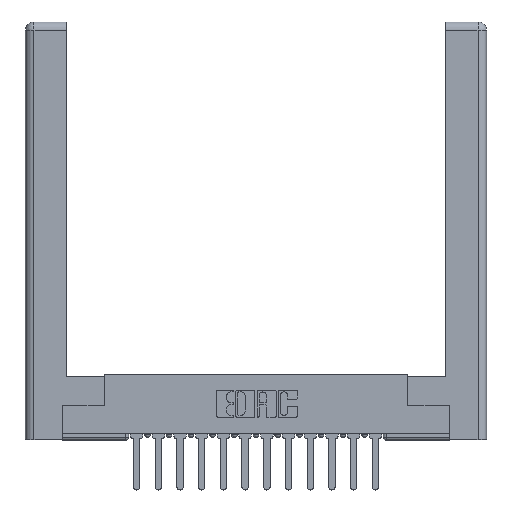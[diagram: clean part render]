
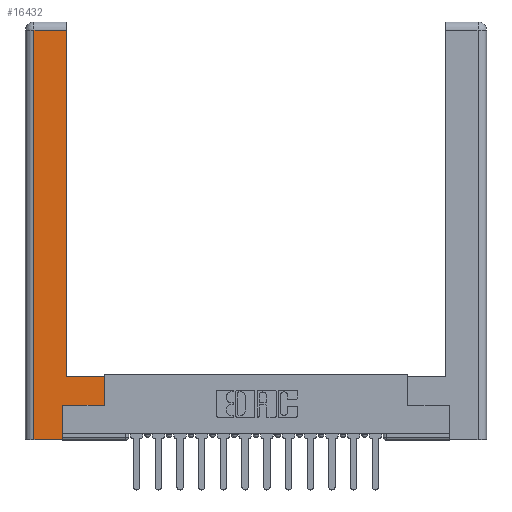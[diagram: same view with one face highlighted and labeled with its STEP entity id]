
A CAD part, top view. The second image highlights one B-rep face of the part: STEP entity #16432.
In plain terms, the highlighted planar face has unit normal (0, 0, 1).
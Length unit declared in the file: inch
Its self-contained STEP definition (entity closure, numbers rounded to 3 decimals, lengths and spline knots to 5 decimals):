
#185 = VECTOR ( 'NONE', #12229, 39.37008 ) ;
#462 = CARTESIAN_POINT ( 'NONE',  ( 0.295, 3., 0. ) ) ;
#764 = VECTOR ( 'NONE', #3290, 39.37008 ) ;
#845 = CARTESIAN_POINT ( 'NONE',  ( 0.265, 0., 0. ) ) ;
#941 = EDGE_CURVE ( 'NONE', #9943, #2166, #15831, .T. ) ;
#943 = ORIENTED_EDGE ( 'NONE', *, *, #9176, .T. ) ;
#1061 = FACE_OUTER_BOUND ( 'NONE', #15952, .T. ) ;
#1888 = DIRECTION ( 'NONE',  ( 0., 1., 0. ) ) ;
#2166 = VERTEX_POINT ( 'NONE', #6446 ) ;
#2201 = LINE ( 'NONE', #7505, #14871 ) ;
#2203 = EDGE_CURVE ( 'NONE', #6351, #10441, #2510, .T. ) ;
#2479 = VECTOR ( 'NONE', #5366, 39.37008 ) ;
#2510 = LINE ( 'NONE', #2670, #2479 ) ;
#2670 = CARTESIAN_POINT ( 'NONE',  ( 0.0615, 0., 0. ) ) ;
#2822 = CARTESIAN_POINT ( 'NONE',  ( 0.0615, 2.94, 0. ) ) ;
#2996 = DIRECTION ( 'NONE',  ( 0., 1., 0. ) ) ;
#3290 = DIRECTION ( 'NONE',  ( 0., 1., 0. ) ) ;
#3300 = EDGE_CURVE ( 'NONE', #8840, #8304, #14601, .T. ) ;
#4397 = EDGE_CURVE ( 'NONE', #10441, #9943, #16046, .T. ) ;
#4528 = CARTESIAN_POINT ( 'NONE',  ( 0.265, 0.245, 0. ) ) ;
#4725 = CARTESIAN_POINT ( 'NONE',  ( 0.565, 0.245, 0. ) ) ;
#5174 = ORIENTED_EDGE ( 'NONE', *, *, #941, .T. ) ;
#5181 = DIRECTION ( 'NONE',  ( -1., 0., 0. ) ) ;
#5227 = ORIENTED_EDGE ( 'NONE', *, *, #2203, .T. ) ;
#5366 = DIRECTION ( 'NONE',  ( 0., -1., 0. ) ) ;
#5504 = VECTOR ( 'NONE', #2996, 39.37008 ) ;
#5516 = CARTESIAN_POINT ( 'NONE',  ( 0.565, 0.45, 0. ) ) ;
#6197 = PLANE ( 'NONE',  #10694 ) ;
#6274 = CARTESIAN_POINT ( 'NONE',  ( 0., 0., 0. ) ) ;
#6351 = VERTEX_POINT ( 'NONE', #2822 ) ;
#6446 = CARTESIAN_POINT ( 'NONE',  ( 0.265, 0.245, 0. ) ) ;
#6498 = LINE ( 'NONE', #462, #5504 ) ;
#6855 = EDGE_CURVE ( 'NONE', #2166, #8840, #11656, .T. ) ;
#7338 = DIRECTION ( 'NONE',  ( -1., 0., 0. ) ) ;
#7436 = CARTESIAN_POINT ( 'NONE',  ( 0.0615, 2.94, 0. ) ) ;
#7505 = CARTESIAN_POINT ( 'NONE',  ( 0.295, 0.45, 0. ) ) ;
#7648 = VECTOR ( 'NONE', #1888, 39.37008 ) ;
#8304 = VERTEX_POINT ( 'NONE', #5516 ) ;
#8419 = ORIENTED_EDGE ( 'NONE', *, *, #4397, .T. ) ;
#8746 = LINE ( 'NONE', #7436, #12140 ) ;
#8840 = VERTEX_POINT ( 'NONE', #4725 ) ;
#9045 = VERTEX_POINT ( 'NONE', #10137 ) ;
#9079 = CARTESIAN_POINT ( 'NONE',  ( 0.565, 0.245, 0. ) ) ;
#9176 = EDGE_CURVE ( 'NONE', #14311, #9045, #6498, .T. ) ;
#9465 = EDGE_CURVE ( 'NONE', #9045, #6351, #8746, .T. ) ;
#9819 = CARTESIAN_POINT ( 'NONE',  ( 0.295, 0.45, 0. ) ) ;
#9943 = VERTEX_POINT ( 'NONE', #13918 ) ;
#9988 = EDGE_CURVE ( 'NONE', #8304, #14311, #2201, .T. ) ;
#10137 = CARTESIAN_POINT ( 'NONE',  ( 0.295, 2.94, 0. ) ) ;
#10363 = CARTESIAN_POINT ( 'NONE',  ( 0.0615, 0., 0. ) ) ;
#10441 = VERTEX_POINT ( 'NONE', #10363 ) ;
#10694 = AXIS2_PLACEMENT_3D ( 'NONE', #6274, #14135, #5181 ) ;
#11656 = LINE ( 'NONE', #9079, #15017 ) ;
#11778 = ORIENTED_EDGE ( 'NONE', *, *, #9988, .T. ) ;
#12140 = VECTOR ( 'NONE', #16399, 39.37008 ) ;
#12229 = DIRECTION ( 'NONE',  ( 1., 0., 0. ) ) ;
#13608 = ORIENTED_EDGE ( 'NONE', *, *, #3300, .T. ) ;
#13723 = ORIENTED_EDGE ( 'NONE', *, *, #9465, .T. ) ;
#13918 = CARTESIAN_POINT ( 'NONE',  ( 0.265, 0., 0. ) ) ;
#14135 = DIRECTION ( 'NONE',  ( 0., 0., -1. ) ) ;
#14193 = DIRECTION ( 'NONE',  ( 1., 0., 0. ) ) ;
#14311 = VERTEX_POINT ( 'NONE', #9819 ) ;
#14601 = LINE ( 'NONE', #14865, #764 ) ;
#14865 = CARTESIAN_POINT ( 'NONE',  ( 0.565, 0.45, 0. ) ) ;
#14871 = VECTOR ( 'NONE', #7338, 39.37008 ) ;
#15017 = VECTOR ( 'NONE', #14193, 39.37008 ) ;
#15339 = ORIENTED_EDGE ( 'NONE', *, *, #6855, .T. ) ;
#15831 = LINE ( 'NONE', #4528, #7648 ) ;
#15952 = EDGE_LOOP ( 'NONE', ( #943, #13723, #5227, #8419, #5174, #15339, #13608, #11778 ) ) ;
#16046 = LINE ( 'NONE', #845, #185 ) ;
#16399 = DIRECTION ( 'NONE',  ( -1., 0., 0. ) ) ;
#16432 = ADVANCED_FACE ( 'NONE', ( #1061 ), #6197, .F. ) ;
